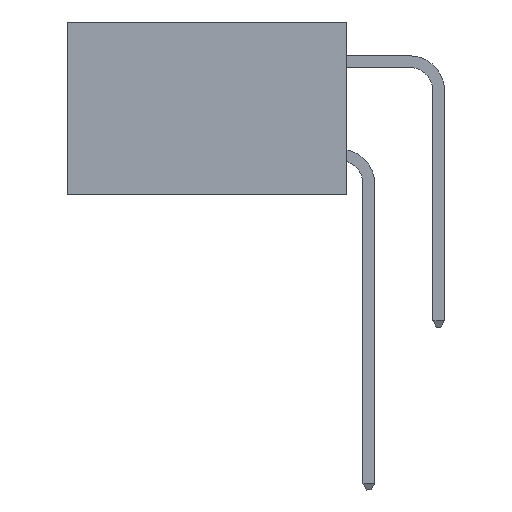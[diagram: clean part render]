
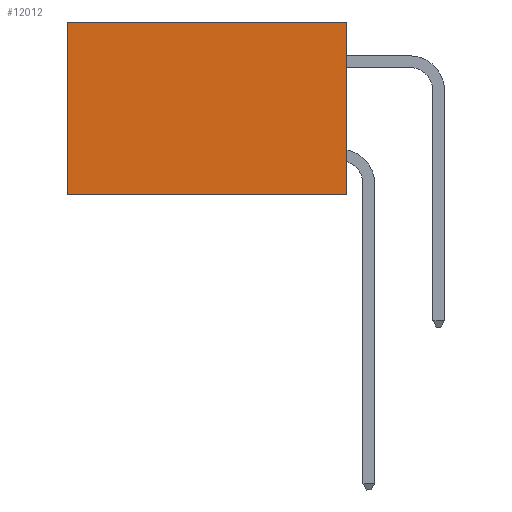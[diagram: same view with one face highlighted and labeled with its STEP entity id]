
A CAD part, left-side view. The second image highlights one B-rep face of the part: STEP entity #12012.
In plain terms, the highlighted planar face has unit normal (-1, 0, 0).
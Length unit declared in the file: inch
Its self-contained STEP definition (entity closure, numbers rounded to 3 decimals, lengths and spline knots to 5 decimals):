
#125 = DIRECTION ( 'NONE',  ( 0., 1., 0. ) ) ;
#255 = EDGE_LOOP ( 'NONE', ( #12963, #7292, #2448, #10059 ) ) ;
#635 = VERTEX_POINT ( 'NONE', #11120 ) ;
#892 = LINE ( 'NONE', #15280, #8987 ) ;
#2013 = CARTESIAN_POINT ( 'NONE',  ( 0.2875, 0.6, 0. ) ) ;
#2448 = ORIENTED_EDGE ( 'NONE', *, *, #20113, .F. ) ;
#2947 = VECTOR ( 'NONE', #5526, 39.37008 ) ;
#4194 = DIRECTION ( 'NONE',  ( 0., 1., 0. ) ) ;
#5526 = DIRECTION ( 'NONE',  ( 0., 0., -1. ) ) ;
#5648 = DIRECTION ( 'NONE',  ( 1., 0., 0. ) ) ;
#6645 = EDGE_CURVE ( 'NONE', #635, #6793, #892, .T. ) ;
#6793 = VERTEX_POINT ( 'NONE', #12470 ) ;
#7022 = LINE ( 'NONE', #13601, #14989 ) ;
#7292 = ORIENTED_EDGE ( 'NONE', *, *, #6645, .F. ) ;
#8229 = CARTESIAN_POINT ( 'NONE',  ( 0.2875, 0., 0. ) ) ;
#8585 = CARTESIAN_POINT ( 'NONE',  ( 0.2875, 0., 0. ) ) ;
#8987 = VECTOR ( 'NONE', #4194, 39.37008 ) ;
#10059 = ORIENTED_EDGE ( 'NONE', *, *, #13074, .T. ) ;
#10251 = CARTESIAN_POINT ( 'NONE',  ( 0.2875, 0.6, 0. ) ) ;
#10385 = PLANE ( 'NONE',  #17732 ) ;
#10455 = FACE_OUTER_BOUND ( 'NONE', #255, .T. ) ;
#11120 = CARTESIAN_POINT ( 'NONE',  ( 0.2875, 0., -0.37 ) ) ;
#11974 = EDGE_CURVE ( 'NONE', #16541, #6793, #15640, .T. ) ;
#12012 = ADVANCED_FACE ( 'NONE', ( #10455 ), #10385, .F. ) ;
#12136 = LINE ( 'NONE', #8229, #19534 ) ;
#12470 = CARTESIAN_POINT ( 'NONE',  ( 0.2875, 0.6, -0.37 ) ) ;
#12963 = ORIENTED_EDGE ( 'NONE', *, *, #11974, .T. ) ;
#13074 = EDGE_CURVE ( 'NONE', #16642, #16541, #12136, .T. ) ;
#13601 = CARTESIAN_POINT ( 'NONE',  ( 0.2875, 0., 0. ) ) ;
#14989 = VECTOR ( 'NONE', #19864, 39.37008 ) ;
#15157 = CARTESIAN_POINT ( 'NONE',  ( 0.2875, 0., 0. ) ) ;
#15280 = CARTESIAN_POINT ( 'NONE',  ( 0.2875, 0., -0.37 ) ) ;
#15640 = LINE ( 'NONE', #10251, #2947 ) ;
#16541 = VERTEX_POINT ( 'NONE', #2013 ) ;
#16642 = VERTEX_POINT ( 'NONE', #8585 ) ;
#16744 = DIRECTION ( 'NONE',  ( 0., 0., -1. ) ) ;
#17732 = AXIS2_PLACEMENT_3D ( 'NONE', #15157, #5648, #16744 ) ;
#19534 = VECTOR ( 'NONE', #125, 39.37008 ) ;
#19864 = DIRECTION ( 'NONE',  ( 0., 0., -1. ) ) ;
#20113 = EDGE_CURVE ( 'NONE', #16642, #635, #7022, .T. ) ;
